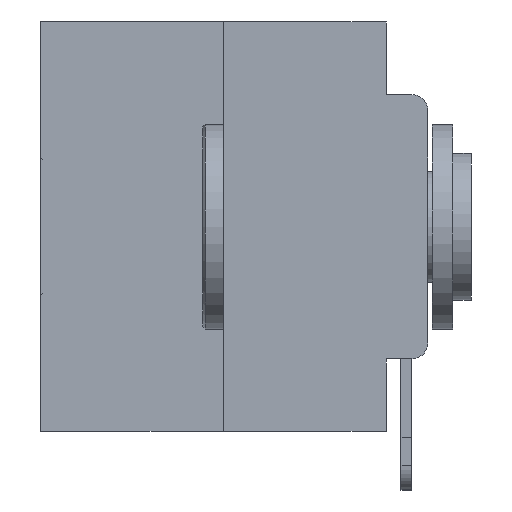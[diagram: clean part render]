
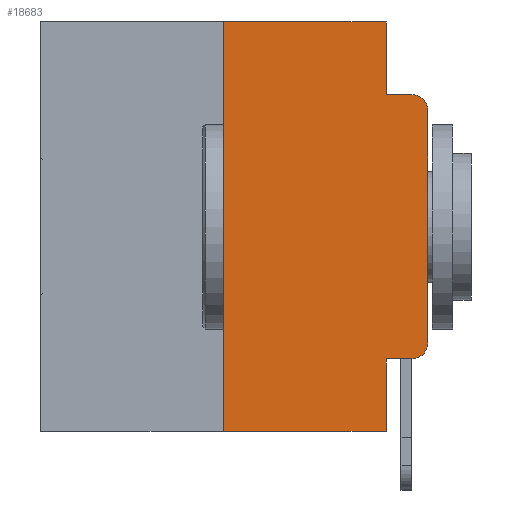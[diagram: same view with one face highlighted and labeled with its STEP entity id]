
A CAD part, left-side view. The second image highlights one B-rep face of the part: STEP entity #18683.
In plain terms, the highlighted planar face has unit normal (-1, 0, 0).
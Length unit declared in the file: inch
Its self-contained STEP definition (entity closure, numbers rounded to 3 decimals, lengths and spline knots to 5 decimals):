
#55 = DIRECTION ( 'NONE',  ( 1., 0., 0. ) ) ;
#651 = CARTESIAN_POINT ( 'NONE',  ( 0., 0.051, -0.0885 ) ) ;
#842 = EDGE_CURVE ( 'NONE', #23201, #24923, #3371, .T. ) ;
#977 = LINE ( 'NONE', #4768, #6055 ) ;
#1276 = EDGE_CURVE ( 'NONE', #23201, #29557, #16677, .T. ) ;
#1966 = VECTOR ( 'NONE', #21399, 39.37008 ) ;
#1979 = CARTESIAN_POINT ( 'NONE',  ( 0., 0.25, 0. ) ) ;
#2076 = DIRECTION ( 'NONE',  ( 0., 0., 1. ) ) ;
#2872 = CARTESIAN_POINT ( 'NONE',  ( 0., 0., 0. ) ) ;
#3371 = LINE ( 'NONE', #1979, #6279 ) ;
#3540 = LINE ( 'NONE', #10013, #13963 ) ;
#3941 = DIRECTION ( 'NONE',  ( 0., 0., -1. ) ) ;
#4434 = VECTOR ( 'NONE', #21164, 39.37008 ) ;
#4742 = EDGE_LOOP ( 'NONE', ( #14422, #25379, #15488, #12649, #27279, #14057, #7367, #9533, #24113, #11582 ) ) ;
#4768 = CARTESIAN_POINT ( 'NONE',  ( 0., 0.051, -0.4115 ) ) ;
#4979 = VERTEX_POINT ( 'NONE', #28941 ) ;
#6055 = VECTOR ( 'NONE', #13992, 39.37008 ) ;
#6279 = VECTOR ( 'NONE', #2076, 39.37008 ) ;
#6847 = VECTOR ( 'NONE', #12073, 39.37008 ) ;
#6905 = CARTESIAN_POINT ( 'NONE',  ( 0., 0.051, 0. ) ) ;
#7033 = PLANE ( 'NONE',  #18415 ) ;
#7367 = ORIENTED_EDGE ( 'NONE', *, *, #1276, .T. ) ;
#7865 = EDGE_CURVE ( 'NONE', #8229, #13352, #12189, .T. ) ;
#8229 = VERTEX_POINT ( 'NONE', #15173 ) ;
#8552 = CARTESIAN_POINT ( 'NONE',  ( 0., 0.051, -0.0885 ) ) ;
#8789 = VERTEX_POINT ( 'NONE', #20107 ) ;
#8811 = VECTOR ( 'NONE', #25307, 39.37008 ) ;
#8815 = CARTESIAN_POINT ( 'NONE',  ( 0., 0.051, -0.5 ) ) ;
#8886 = EDGE_CURVE ( 'NONE', #13764, #29557, #21106, .T. ) ;
#9075 = DIRECTION ( 'NONE',  ( 0., 0., -1. ) ) ;
#9526 = LINE ( 'NONE', #13362, #8811 ) ;
#9533 = ORIENTED_EDGE ( 'NONE', *, *, #8886, .F. ) ;
#9698 = CARTESIAN_POINT ( 'NONE',  ( 0., 0.473, -0.5 ) ) ;
#9907 = DIRECTION ( 'NONE',  ( 0., -1., 0. ) ) ;
#10013 = CARTESIAN_POINT ( 'NONE',  ( 0., 0.473, 0. ) ) ;
#11014 = LINE ( 'NONE', #651, #1966 ) ;
#11548 = DIRECTION ( 'NONE',  ( 0., 0., -1. ) ) ;
#11582 = ORIENTED_EDGE ( 'NONE', *, *, #26426, .T. ) ;
#11586 = DIRECTION ( 'NONE',  ( 0., 0., -1. ) ) ;
#11839 = VERTEX_POINT ( 'NONE', #8552 ) ;
#12073 = DIRECTION ( 'NONE',  ( 0., 0., 1. ) ) ;
#12153 = EDGE_CURVE ( 'NONE', #11839, #13352, #11014, .T. ) ;
#12189 = CIRCLE ( 'NONE', #24235, 0.02 ) ;
#12649 = ORIENTED_EDGE ( 'NONE', *, *, #27738, .F. ) ;
#13352 = VERTEX_POINT ( 'NONE', #23779 ) ;
#13362 = CARTESIAN_POINT ( 'NONE',  ( 0., 0.051, 0. ) ) ;
#13442 = CARTESIAN_POINT ( 'NONE',  ( 0., 0.051, -0.4115 ) ) ;
#13764 = VERTEX_POINT ( 'NONE', #13442 ) ;
#13963 = VECTOR ( 'NONE', #9907, 39.37008 ) ;
#13992 = DIRECTION ( 'NONE',  ( 0., -1., 0. ) ) ;
#14057 = ORIENTED_EDGE ( 'NONE', *, *, #842, .F. ) ;
#14359 = FACE_OUTER_BOUND ( 'NONE', #4742, .T. ) ;
#14422 = ORIENTED_EDGE ( 'NONE', *, *, #18746, .T. ) ;
#14508 = CARTESIAN_POINT ( 'NONE',  ( 0., 0., -0.3915 ) ) ;
#14690 = AXIS2_PLACEMENT_3D ( 'NONE', #27044, #24919, #3941 ) ;
#15173 = CARTESIAN_POINT ( 'NONE',  ( 0., 0., -0.1085 ) ) ;
#15488 = ORIENTED_EDGE ( 'NONE', *, *, #12153, .F. ) ;
#16015 = EDGE_CURVE ( 'NONE', #13764, #4979, #977, .T. ) ;
#16677 = LINE ( 'NONE', #9698, #4434 ) ;
#17703 = CARTESIAN_POINT ( 'NONE',  ( 0., 0.25, 0. ) ) ;
#18415 = AXIS2_PLACEMENT_3D ( 'NONE', #25303, #55, #11586 ) ;
#18683 = ADVANCED_FACE ( 'NONE', ( #14359 ), #7033, .F. ) ;
#18746 = EDGE_CURVE ( 'NONE', #20025, #8229, #22324, .T. ) ;
#19512 = EDGE_CURVE ( 'NONE', #24923, #8789, #3540, .T. ) ;
#20025 = VERTEX_POINT ( 'NONE', #14508 ) ;
#20107 = CARTESIAN_POINT ( 'NONE',  ( 0., 0.051, 0. ) ) ;
#21106 = LINE ( 'NONE', #6905, #22214 ) ;
#21164 = DIRECTION ( 'NONE',  ( 0., -1., 0. ) ) ;
#21399 = DIRECTION ( 'NONE',  ( 0., -1., 0. ) ) ;
#22214 = VECTOR ( 'NONE', #11548, 39.37008 ) ;
#22324 = LINE ( 'NONE', #2872, #6847 ) ;
#22474 = CARTESIAN_POINT ( 'NONE',  ( 0., 0.02, -0.1085 ) ) ;
#22803 = CARTESIAN_POINT ( 'NONE',  ( 0., 0.25, -0.5 ) ) ;
#23201 = VERTEX_POINT ( 'NONE', #22803 ) ;
#23779 = CARTESIAN_POINT ( 'NONE',  ( 0., 0.02, -0.0885 ) ) ;
#24113 = ORIENTED_EDGE ( 'NONE', *, *, #16015, .T. ) ;
#24235 = AXIS2_PLACEMENT_3D ( 'NONE', #22474, #29711, #9075 ) ;
#24428 = CIRCLE ( 'NONE', #14690, 0.02 ) ;
#24919 = DIRECTION ( 'NONE',  ( -1., 0., 0. ) ) ;
#24923 = VERTEX_POINT ( 'NONE', #17703 ) ;
#25303 = CARTESIAN_POINT ( 'NONE',  ( 0., 0.473, 0. ) ) ;
#25307 = DIRECTION ( 'NONE',  ( 0., 0., -1. ) ) ;
#25379 = ORIENTED_EDGE ( 'NONE', *, *, #7865, .T. ) ;
#26426 = EDGE_CURVE ( 'NONE', #4979, #20025, #24428, .T. ) ;
#27044 = CARTESIAN_POINT ( 'NONE',  ( 0., 0.02, -0.3915 ) ) ;
#27279 = ORIENTED_EDGE ( 'NONE', *, *, #19512, .F. ) ;
#27738 = EDGE_CURVE ( 'NONE', #8789, #11839, #9526, .T. ) ;
#28941 = CARTESIAN_POINT ( 'NONE',  ( 0., 0.02, -0.4115 ) ) ;
#29557 = VERTEX_POINT ( 'NONE', #8815 ) ;
#29711 = DIRECTION ( 'NONE',  ( -1., 0., 0. ) ) ;
